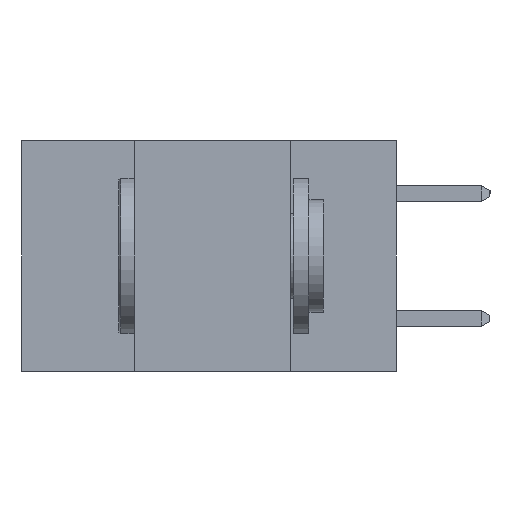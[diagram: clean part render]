
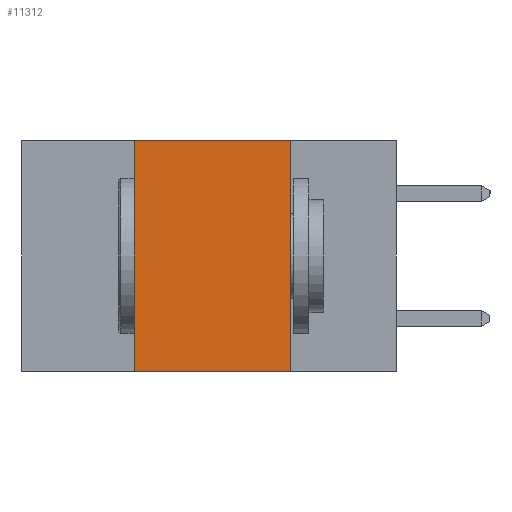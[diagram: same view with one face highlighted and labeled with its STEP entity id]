
A CAD part, left-side view. The second image highlights one B-rep face of the part: STEP entity #11312.
In plain terms, the highlighted planar face has unit normal (-1, 0, 0).
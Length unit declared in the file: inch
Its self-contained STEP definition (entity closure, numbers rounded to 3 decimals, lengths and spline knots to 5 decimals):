
#333 = DIRECTION ( 'NONE',  ( 0., -1., 0. ) ) ;
#369 = CARTESIAN_POINT ( 'NONE',  ( 0., 0.42, -0.37 ) ) ;
#701 = ORIENTED_EDGE ( 'NONE', *, *, #4577, .F. ) ;
#1646 = DIRECTION ( 'NONE',  ( 0., 0., 1. ) ) ;
#2570 = VECTOR ( 'NONE', #8550, 39.37008 ) ;
#3096 = CARTESIAN_POINT ( 'NONE',  ( 0., 0.6, 0. ) ) ;
#3478 = DIRECTION ( 'NONE',  ( 0., 0., -1. ) ) ;
#3683 = CARTESIAN_POINT ( 'NONE',  ( 0., 0.17, -0.37 ) ) ;
#4577 = EDGE_CURVE ( 'NONE', #17989, #21164, #19547, .T. ) ;
#5529 = LINE ( 'NONE', #7126, #17507 ) ;
#6126 = AXIS2_PLACEMENT_3D ( 'NONE', #3096, #19282, #3478 ) ;
#7126 = CARTESIAN_POINT ( 'NONE',  ( 0., 0.6, -0.37 ) ) ;
#8550 = DIRECTION ( 'NONE',  ( 0., 0., -1. ) ) ;
#10144 = CARTESIAN_POINT ( 'NONE',  ( 0., 0.6, 0. ) ) ;
#10667 = CARTESIAN_POINT ( 'NONE',  ( 0., 0.42, 0. ) ) ;
#10735 = ORIENTED_EDGE ( 'NONE', *, *, #22778, .F. ) ;
#11312 = ADVANCED_FACE ( 'NONE', ( #21365 ), #11320, .F. ) ;
#11320 = PLANE ( 'NONE',  #6126 ) ;
#11706 = CARTESIAN_POINT ( 'NONE',  ( 0., 0.42, -0.37 ) ) ;
#12207 = LINE ( 'NONE', #22512, #2570 ) ;
#13510 = CARTESIAN_POINT ( 'NONE',  ( 0., 0.17, 0. ) ) ;
#13769 = EDGE_CURVE ( 'NONE', #21164, #20011, #22139, .T. ) ;
#16166 = VECTOR ( 'NONE', #333, 39.37008 ) ;
#17252 = EDGE_CURVE ( 'NONE', #17989, #23149, #5529, .T. ) ;
#17489 = ORIENTED_EDGE ( 'NONE', *, *, #17252, .T. ) ;
#17507 = VECTOR ( 'NONE', #23035, 39.37008 ) ;
#17989 = VERTEX_POINT ( 'NONE', #369 ) ;
#19282 = DIRECTION ( 'NONE',  ( 1., 0., 0. ) ) ;
#19547 = LINE ( 'NONE', #11706, #20571 ) ;
#20011 = VERTEX_POINT ( 'NONE', #13510 ) ;
#20571 = VECTOR ( 'NONE', #1646, 39.37008 ) ;
#21164 = VERTEX_POINT ( 'NONE', #10667 ) ;
#21365 = FACE_OUTER_BOUND ( 'NONE', #24906, .T. ) ;
#22139 = LINE ( 'NONE', #10144, #16166 ) ;
#22512 = CARTESIAN_POINT ( 'NONE',  ( 0., 0.17, -0.37 ) ) ;
#22778 = EDGE_CURVE ( 'NONE', #20011, #23149, #12207, .T. ) ;
#23035 = DIRECTION ( 'NONE',  ( 0., -1., 0. ) ) ;
#23149 = VERTEX_POINT ( 'NONE', #3683 ) ;
#23915 = ORIENTED_EDGE ( 'NONE', *, *, #13769, .F. ) ;
#24906 = EDGE_LOOP ( 'NONE', ( #10735, #23915, #701, #17489 ) ) ;
